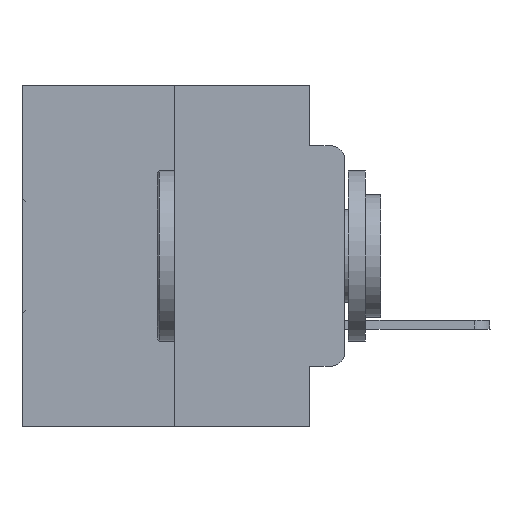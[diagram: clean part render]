
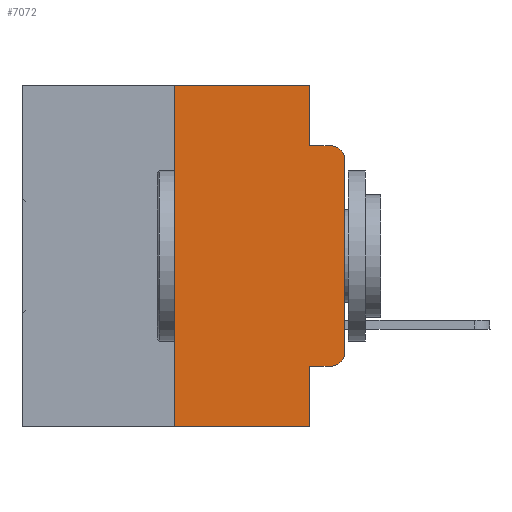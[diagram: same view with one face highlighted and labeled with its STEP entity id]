
A CAD part, left-side view. The second image highlights one B-rep face of the part: STEP entity #7072.
In plain terms, the highlighted planar face has unit normal (-1, 0, 0).
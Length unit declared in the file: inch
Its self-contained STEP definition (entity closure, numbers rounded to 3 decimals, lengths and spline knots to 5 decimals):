
#560 = ORIENTED_EDGE ( 'NONE', *, *, #9510, .T. ) ;
#583 = LINE ( 'NONE', #10402, #12491 ) ;
#635 = DIRECTION ( 'NONE',  ( 0., 0., -1. ) ) ;
#1092 = FACE_OUTER_BOUND ( 'NONE', #18349, .T. ) ;
#1103 = ORIENTED_EDGE ( 'NONE', *, *, #3044, .T. ) ;
#1147 = LINE ( 'NONE', #28417, #5526 ) ;
#1413 = CARTESIAN_POINT ( 'NONE',  ( 0., 0., -0.1085 ) ) ;
#1567 = ORIENTED_EDGE ( 'NONE', *, *, #2661, .F. ) ;
#2310 = EDGE_CURVE ( 'NONE', #10634, #8843, #2715, .T. ) ;
#2456 = DIRECTION ( 'NONE',  ( 0., 0., -1. ) ) ;
#2661 = EDGE_CURVE ( 'NONE', #18890, #22869, #16713, .T. ) ;
#2715 = LINE ( 'NONE', #27244, #3699 ) ;
#3044 = EDGE_CURVE ( 'NONE', #19351, #22869, #16787, .T. ) ;
#3084 = ORIENTED_EDGE ( 'NONE', *, *, #21222, .T. ) ;
#3481 = VECTOR ( 'NONE', #18521, 39.37008 ) ;
#3699 = VECTOR ( 'NONE', #12543, 39.37008 ) ;
#4163 = EDGE_CURVE ( 'NONE', #25905, #18890, #9121, .T. ) ;
#4316 = CIRCLE ( 'NONE', #22329, 0.02 ) ;
#5526 = VECTOR ( 'NONE', #23219, 39.37008 ) ;
#7072 = ADVANCED_FACE ( 'NONE', ( #1092 ), #20903, .F. ) ;
#7096 = DIRECTION ( 'NONE',  ( -1., 0., 0. ) ) ;
#7329 = ORIENTED_EDGE ( 'NONE', *, *, #2310, .T. ) ;
#7570 = CARTESIAN_POINT ( 'NONE',  ( 0., 0.051, 0. ) ) ;
#8194 = DIRECTION ( 'NONE',  ( 1., 0., 0. ) ) ;
#8630 = VERTEX_POINT ( 'NONE', #12473 ) ;
#8843 = VERTEX_POINT ( 'NONE', #28604 ) ;
#8853 = CARTESIAN_POINT ( 'NONE',  ( 0., 0.473, 0. ) ) ;
#9121 = LINE ( 'NONE', #28656, #12823 ) ;
#9510 = EDGE_CURVE ( 'NONE', #28331, #22815, #583, .T. ) ;
#10402 = CARTESIAN_POINT ( 'NONE',  ( 0., 0.051, -0.4115 ) ) ;
#10634 = VERTEX_POINT ( 'NONE', #21911 ) ;
#10752 = CARTESIAN_POINT ( 'NONE',  ( 0., 0.02, -0.0885 ) ) ;
#11557 = CARTESIAN_POINT ( 'NONE',  ( 0., 0.051, 0. ) ) ;
#11593 = VECTOR ( 'NONE', #28990, 39.37008 ) ;
#11905 = CARTESIAN_POINT ( 'NONE',  ( 0., 0.02, -0.3915 ) ) ;
#12097 = CARTESIAN_POINT ( 'NONE',  ( 0., 0.02, -0.1085 ) ) ;
#12201 = EDGE_CURVE ( 'NONE', #22815, #25926, #4316, .T. ) ;
#12473 = CARTESIAN_POINT ( 'NONE',  ( 0., 0.25, 0. ) ) ;
#12491 = VECTOR ( 'NONE', #20250, 39.37008 ) ;
#12543 = DIRECTION ( 'NONE',  ( 0., -1., 0. ) ) ;
#12823 = VECTOR ( 'NONE', #635, 39.37008 ) ;
#13354 = ORIENTED_EDGE ( 'NONE', *, *, #15198, .F. ) ;
#13493 = ORIENTED_EDGE ( 'NONE', *, *, #23724, .F. ) ;
#14592 = LINE ( 'NONE', #24912, #23389 ) ;
#15198 = EDGE_CURVE ( 'NONE', #28331, #8843, #18672, .T. ) ;
#15691 = CARTESIAN_POINT ( 'NONE',  ( 0., 0.051, -0.0885 ) ) ;
#15980 = LINE ( 'NONE', #8853, #21671 ) ;
#16177 = ORIENTED_EDGE ( 'NONE', *, *, #29575, .F. ) ;
#16272 = CARTESIAN_POINT ( 'NONE',  ( 0., 0.051, -0.4115 ) ) ;
#16282 = AXIS2_PLACEMENT_3D ( 'NONE', #25432, #8194, #18172 ) ;
#16713 = LINE ( 'NONE', #29146, #11593 ) ;
#16787 = CIRCLE ( 'NONE', #27601, 0.02 ) ;
#16800 = DIRECTION ( 'NONE',  ( -1., 0., 0. ) ) ;
#17094 = DIRECTION ( 'NONE',  ( 0., 0., -1. ) ) ;
#17407 = CARTESIAN_POINT ( 'NONE',  ( 0., 0., -0.3915 ) ) ;
#18172 = DIRECTION ( 'NONE',  ( 0., 0., -1. ) ) ;
#18349 = EDGE_LOOP ( 'NONE', ( #3084, #1103, #1567, #22878, #16177, #13493, #7329, #13354, #560, #20523 ) ) ;
#18521 = DIRECTION ( 'NONE',  ( 0., 0., -1. ) ) ;
#18672 = LINE ( 'NONE', #11557, #3481 ) ;
#18890 = VERTEX_POINT ( 'NONE', #15691 ) ;
#19351 = VERTEX_POINT ( 'NONE', #1413 ) ;
#20250 = DIRECTION ( 'NONE',  ( 0., -1., 0. ) ) ;
#20523 = ORIENTED_EDGE ( 'NONE', *, *, #12201, .T. ) ;
#20903 = PLANE ( 'NONE',  #16282 ) ;
#21222 = EDGE_CURVE ( 'NONE', #25926, #19351, #14592, .T. ) ;
#21671 = VECTOR ( 'NONE', #30839, 39.37008 ) ;
#21911 = CARTESIAN_POINT ( 'NONE',  ( 0., 0.25, -0.5 ) ) ;
#22172 = DIRECTION ( 'NONE',  ( 0., 0., 1. ) ) ;
#22329 = AXIS2_PLACEMENT_3D ( 'NONE', #11905, #7096, #17094 ) ;
#22815 = VERTEX_POINT ( 'NONE', #28033 ) ;
#22869 = VERTEX_POINT ( 'NONE', #10752 ) ;
#22878 = ORIENTED_EDGE ( 'NONE', *, *, #4163, .F. ) ;
#23219 = DIRECTION ( 'NONE',  ( 0., 0., 1. ) ) ;
#23389 = VECTOR ( 'NONE', #22172, 39.37008 ) ;
#23724 = EDGE_CURVE ( 'NONE', #10634, #8630, #1147, .T. ) ;
#24912 = CARTESIAN_POINT ( 'NONE',  ( 0., 0., 0. ) ) ;
#25432 = CARTESIAN_POINT ( 'NONE',  ( 0., 0.473, 0. ) ) ;
#25905 = VERTEX_POINT ( 'NONE', #7570 ) ;
#25926 = VERTEX_POINT ( 'NONE', #17407 ) ;
#27244 = CARTESIAN_POINT ( 'NONE',  ( 0., 0.473, -0.5 ) ) ;
#27601 = AXIS2_PLACEMENT_3D ( 'NONE', #12097, #16800, #2456 ) ;
#28033 = CARTESIAN_POINT ( 'NONE',  ( 0., 0.02, -0.4115 ) ) ;
#28331 = VERTEX_POINT ( 'NONE', #16272 ) ;
#28417 = CARTESIAN_POINT ( 'NONE',  ( 0., 0.25, 0. ) ) ;
#28604 = CARTESIAN_POINT ( 'NONE',  ( 0., 0.051, -0.5 ) ) ;
#28656 = CARTESIAN_POINT ( 'NONE',  ( 0., 0.051, 0. ) ) ;
#28990 = DIRECTION ( 'NONE',  ( 0., -1., 0. ) ) ;
#29146 = CARTESIAN_POINT ( 'NONE',  ( 0., 0.051, -0.0885 ) ) ;
#29575 = EDGE_CURVE ( 'NONE', #8630, #25905, #15980, .T. ) ;
#30839 = DIRECTION ( 'NONE',  ( 0., -1., 0. ) ) ;
